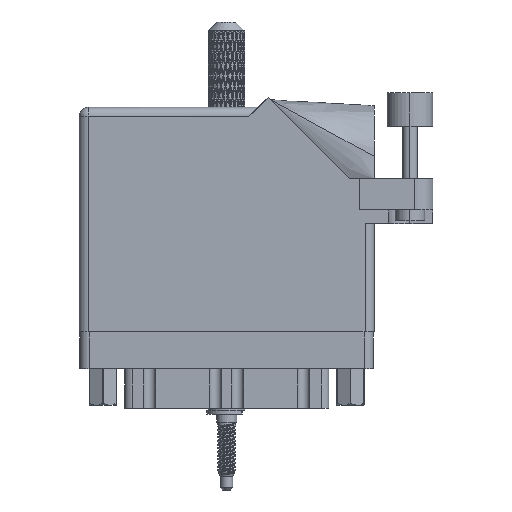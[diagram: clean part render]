
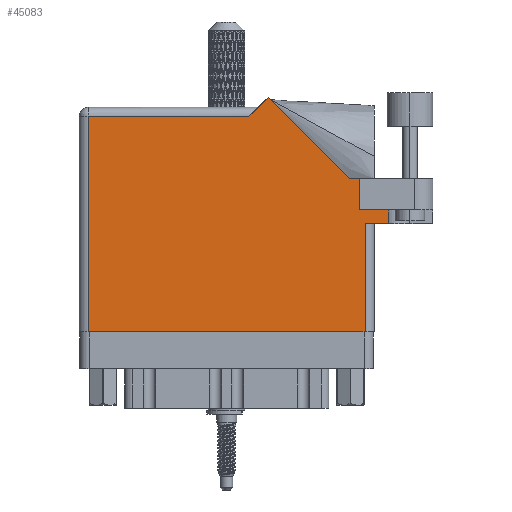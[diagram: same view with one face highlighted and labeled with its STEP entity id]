
A CAD part, front view. The second image highlights one B-rep face of the part: STEP entity #45083.
In plain terms, the highlighted face is planar.
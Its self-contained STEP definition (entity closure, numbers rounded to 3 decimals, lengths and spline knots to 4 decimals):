
#2612 = VECTOR ( 'NONE', #62983, 39.3701 ) ;
#3839 = VECTOR ( 'NONE', #35361, 39.3701 ) ;
#4041 = EDGE_CURVE ( 'NONE', #59778, #91101, #48461, .T. ) ;
#4635 = VECTOR ( 'NONE', #36685, 39.3701 ) ;
#5722 = VERTEX_POINT ( 'NONE', #54931 ) ;
#5801 = EDGE_LOOP ( 'NONE', ( #17317, #20538, #98854, #53761, #107173, #64032, #6628, #94603, #96935, #27990, #48399 ) ) ;
#6628 = ORIENTED_EDGE ( 'NONE', *, *, #111002, .T. ) ;
#7108 = LINE ( 'NONE', #43877, #28264 ) ;
#8597 = FACE_OUTER_BOUND ( 'NONE', #5801, .T. ) ;
#9924 = VERTEX_POINT ( 'NONE', #71334 ) ;
#11280 = VECTOR ( 'NONE', #21465, 39.3701 ) ;
#11821 = CARTESIAN_POINT ( 'NONE',  ( 2.41, 1.044, 0. ) ) ;
#14979 = VECTOR ( 'NONE', #69656, 39.3701 ) ;
#16419 = CARTESIAN_POINT ( 'NONE',  ( 1.91, 0.831, 0. ) ) ;
#16930 = LINE ( 'NONE', #80647, #106656 ) ;
#17317 = ORIENTED_EDGE ( 'NONE', *, *, #29506, .T. ) ;
#17868 = CARTESIAN_POINT ( 'NONE',  ( 2.1115, 0.737, 0. ) ) ;
#18965 = VERTEX_POINT ( 'NONE', #78383 ) ;
#20538 = ORIENTED_EDGE ( 'NONE', *, *, #111963, .T. ) ;
#20845 = VECTOR ( 'NONE', #58945, 39.3701 ) ;
#21465 = DIRECTION ( 'NONE',  ( 0., -1., 0. ) ) ;
#22506 = VERTEX_POINT ( 'NONE', #17868 ) ;
#24986 = DIRECTION ( 'NONE',  ( 1., 0., 0. ) ) ;
#25614 = LINE ( 'NONE', #16419, #3839 ) ;
#25731 = VERTEX_POINT ( 'NONE', #81522 ) ;
#26106 = CARTESIAN_POINT ( 'NONE',  ( 0., 0., 0. ) ) ;
#27247 = DIRECTION ( 'NONE',  ( 0., 1., 0. ) ) ;
#27990 = ORIENTED_EDGE ( 'NONE', *, *, #84647, .T. ) ;
#28264 = VECTOR ( 'NONE', #42155, 39.3701 ) ;
#29506 = EDGE_CURVE ( 'NONE', #91101, #18965, #111134, .T. ) ;
#34160 = VECTOR ( 'NONE', #24986, 39.3701 ) ;
#35361 = DIRECTION ( 'NONE',  ( 1., 0., 0. ) ) ;
#35586 = EDGE_CURVE ( 'NONE', #92060, #9924, #16930, .T. ) ;
#36685 = DIRECTION ( 'NONE',  ( 1., 0., 0. ) ) ;
#42155 = DIRECTION ( 'NONE',  ( 0., 1., 0. ) ) ;
#43877 = CARTESIAN_POINT ( 'NONE',  ( 1.948, 0.737, 0. ) ) ;
#44758 = LINE ( 'NONE', #53932, #4635 ) ;
#45083 = ADVANCED_FACE ( 'NONE', ( #8597 ), #102817, .F. ) ;
#45285 = VERTEX_POINT ( 'NONE', #62381 ) ;
#45396 = DIRECTION ( 'NONE',  ( -0.707, 0.707, 0. ) ) ;
#45546 = EDGE_CURVE ( 'NONE', #25731, #22506, #69841, .T. ) ;
#46555 = EDGE_CURVE ( 'NONE', #5722, #75666, #89049, .T. ) ;
#46591 = VECTOR ( 'NONE', #45396, 39.3701 ) ;
#48399 = ORIENTED_EDGE ( 'NONE', *, *, #4041, .T. ) ;
#48461 = LINE ( 'NONE', #83506, #11280 ) ;
#51154 = DIRECTION ( 'NONE',  ( -1., 0., 0. ) ) ;
#51276 = CARTESIAN_POINT ( 'NONE',  ( 1.217, 1.53, 0. ) ) ;
#52149 = CARTESIAN_POINT ( 'NONE',  ( 1.2877, 1.6007, 0. ) ) ;
#52273 = DIRECTION ( 'NONE',  ( 0., 0., -1. ) ) ;
#53761 = ORIENTED_EDGE ( 'NONE', *, *, #45546, .F. ) ;
#53932 = CARTESIAN_POINT ( 'NONE',  ( 2.01, 0.737, 0. ) ) ;
#54931 = CARTESIAN_POINT ( 'NONE',  ( 1.8444, 1.044, 0. ) ) ;
#58945 = DIRECTION ( 'NONE',  ( 0., -1., 0. ) ) ;
#59778 = VERTEX_POINT ( 'NONE', #69635 ) ;
#62381 = CARTESIAN_POINT ( 'NONE',  ( 1.948, 0.737, 0. ) ) ;
#62983 = DIRECTION ( 'NONE',  ( -1., 0., 0. ) ) ;
#64032 = ORIENTED_EDGE ( 'NONE', *, *, #35586, .T. ) ;
#69635 = CARTESIAN_POINT ( 'NONE',  ( 0.062, 1.468, 0. ) ) ;
#69656 = DIRECTION ( 'NONE',  ( -0.707, -0.707, 0. ) ) ;
#69841 = LINE ( 'NONE', #95139, #20845 ) ;
#70969 = DIRECTION ( 'NONE',  ( -1., 0., 0. ) ) ;
#71334 = CARTESIAN_POINT ( 'NONE',  ( 1.91, 1.044, 0. ) ) ;
#72321 = EDGE_CURVE ( 'NONE', #92060, #25731, #25614, .T. ) ;
#73645 = EDGE_CURVE ( 'NONE', #75666, #94563, #96069, .T. ) ;
#75666 = VERTEX_POINT ( 'NONE', #52149 ) ;
#78383 = CARTESIAN_POINT ( 'NONE',  ( 1.948, 0., 0. ) ) ;
#79556 = LINE ( 'NONE', #80688, #103636 ) ;
#80647 = CARTESIAN_POINT ( 'NONE',  ( 1.91, 0.831, 0. ) ) ;
#80688 = CARTESIAN_POINT ( 'NONE',  ( 0., 1.468, 0. ) ) ;
#81522 = CARTESIAN_POINT ( 'NONE',  ( 2.1115, 0.831, 0. ) ) ;
#83506 = CARTESIAN_POINT ( 'NONE',  ( 0.062, 0., 0. ) ) ;
#84647 = EDGE_CURVE ( 'NONE', #94563, #59778, #79556, .T. ) ;
#86138 = EDGE_CURVE ( 'NONE', #45285, #22506, #44758, .T. ) ;
#89049 = LINE ( 'NONE', #105720, #46591 ) ;
#90264 = CARTESIAN_POINT ( 'NONE',  ( 0.062, 0., 0. ) ) ;
#91101 = VERTEX_POINT ( 'NONE', #90264 ) ;
#92060 = VERTEX_POINT ( 'NONE', #104715 ) ;
#94563 = VERTEX_POINT ( 'NONE', #97134 ) ;
#94603 = ORIENTED_EDGE ( 'NONE', *, *, #46555, .T. ) ;
#95139 = CARTESIAN_POINT ( 'NONE',  ( 2.1115, 1.1618, 0. ) ) ;
#96069 = LINE ( 'NONE', #51276, #14979 ) ;
#96935 = ORIENTED_EDGE ( 'NONE', *, *, #73645, .T. ) ;
#97134 = CARTESIAN_POINT ( 'NONE',  ( 1.155, 1.468, 0. ) ) ;
#98854 = ORIENTED_EDGE ( 'NONE', *, *, #86138, .T. ) ;
#99756 = AXIS2_PLACEMENT_3D ( 'NONE', #105108, #52273, #51154 ) ;
#102817 = PLANE ( 'NONE',  #99756 ) ;
#103636 = VECTOR ( 'NONE', #70969, 39.3701 ) ;
#104715 = CARTESIAN_POINT ( 'NONE',  ( 1.91, 0.831, 0. ) ) ;
#105108 = CARTESIAN_POINT ( 'NONE',  ( 0., 1.53, 0. ) ) ;
#105720 = CARTESIAN_POINT ( 'NONE',  ( 1.8444, 1.044, 0. ) ) ;
#106656 = VECTOR ( 'NONE', #27247, 39.3701 ) ;
#107173 = ORIENTED_EDGE ( 'NONE', *, *, #72321, .F. ) ;
#108863 = LINE ( 'NONE', #11821, #2612 ) ;
#111002 = EDGE_CURVE ( 'NONE', #9924, #5722, #108863, .T. ) ;
#111134 = LINE ( 'NONE', #26106, #34160 ) ;
#111963 = EDGE_CURVE ( 'NONE', #18965, #45285, #7108, .T. ) ;
